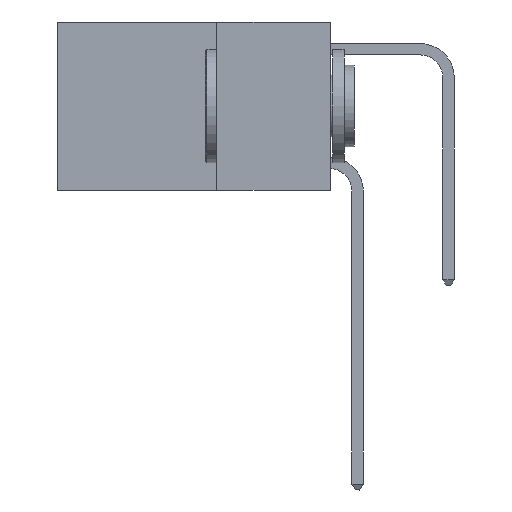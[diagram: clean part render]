
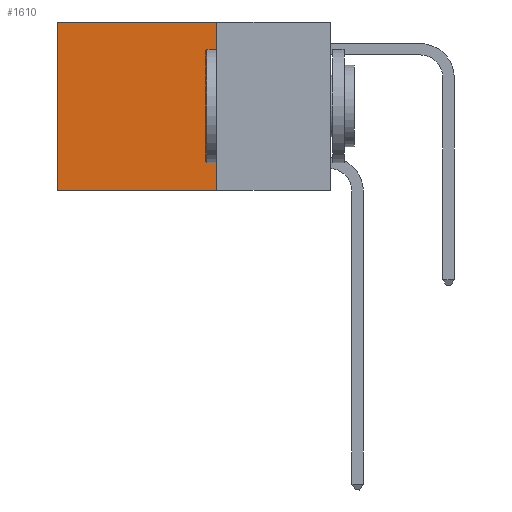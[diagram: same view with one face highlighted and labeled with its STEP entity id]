
A CAD part, left-side view. The second image highlights one B-rep face of the part: STEP entity #1610.
In plain terms, the highlighted planar face has unit normal (-1, 0, 0).
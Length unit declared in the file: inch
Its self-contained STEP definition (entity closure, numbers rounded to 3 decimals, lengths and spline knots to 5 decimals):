
#457 = CARTESIAN_POINT ( 'NONE',  ( 0.2625, 0.25, 0. ) ) ;
#1170 = VECTOR ( 'NONE', #5583, 39.37008 ) ;
#1394 = VERTEX_POINT ( 'NONE', #8471 ) ;
#1610 = ADVANCED_FACE ( 'NONE', ( #7768 ), #3757, .F. ) ;
#2112 = LINE ( 'NONE', #3383, #6817 ) ;
#2234 = VERTEX_POINT ( 'NONE', #4405 ) ;
#2416 = LINE ( 'NONE', #10931, #7415 ) ;
#2614 = CARTESIAN_POINT ( 'NONE',  ( 0.2625, 0.25, -0.37 ) ) ;
#3239 = LINE ( 'NONE', #2614, #11157 ) ;
#3383 = CARTESIAN_POINT ( 'NONE',  ( 0.2625, 0.6, 0. ) ) ;
#3575 = VERTEX_POINT ( 'NONE', #6453 ) ;
#3626 = DIRECTION ( 'NONE',  ( 0., 0., -1. ) ) ;
#3711 = DIRECTION ( 'NONE',  ( 1., 0., 0. ) ) ;
#3733 = CARTESIAN_POINT ( 'NONE',  ( 0.2625, 0.25, 0. ) ) ;
#3740 = CARTESIAN_POINT ( 'NONE',  ( 0.2625, 0.6, 0. ) ) ;
#3757 = PLANE ( 'NONE',  #8220 ) ;
#3978 = EDGE_LOOP ( 'NONE', ( #6916, #9011, #5839, #8820 ) ) ;
#4405 = CARTESIAN_POINT ( 'NONE',  ( 0.2625, 0.25, -0.37 ) ) ;
#4704 = EDGE_CURVE ( 'NONE', #1394, #2234, #11423, .T. ) ;
#4854 = DIRECTION ( 'NONE',  ( 0., 1., 0. ) ) ;
#5583 = DIRECTION ( 'NONE',  ( 0., 0., -1. ) ) ;
#5839 = ORIENTED_EDGE ( 'NONE', *, *, #4704, .F. ) ;
#6453 = CARTESIAN_POINT ( 'NONE',  ( 0.2625, 0.6, -0.37 ) ) ;
#6817 = VECTOR ( 'NONE', #11316, 39.37008 ) ;
#6916 = ORIENTED_EDGE ( 'NONE', *, *, #11519, .T. ) ;
#7415 = VECTOR ( 'NONE', #11876, 39.37008 ) ;
#7768 = FACE_OUTER_BOUND ( 'NONE', #3978, .T. ) ;
#8220 = AXIS2_PLACEMENT_3D ( 'NONE', #3733, #3711, #3626 ) ;
#8471 = CARTESIAN_POINT ( 'NONE',  ( 0.2625, 0.25, 0. ) ) ;
#8820 = ORIENTED_EDGE ( 'NONE', *, *, #11893, .T. ) ;
#9011 = ORIENTED_EDGE ( 'NONE', *, *, #10482, .F. ) ;
#9878 = VERTEX_POINT ( 'NONE', #3740 ) ;
#10482 = EDGE_CURVE ( 'NONE', #2234, #3575, #3239, .T. ) ;
#10931 = CARTESIAN_POINT ( 'NONE',  ( 0.2625, 0.25, 0. ) ) ;
#11157 = VECTOR ( 'NONE', #4854, 39.37008 ) ;
#11316 = DIRECTION ( 'NONE',  ( 0., 0., -1. ) ) ;
#11423 = LINE ( 'NONE', #457, #1170 ) ;
#11519 = EDGE_CURVE ( 'NONE', #9878, #3575, #2112, .T. ) ;
#11876 = DIRECTION ( 'NONE',  ( 0., 1., 0. ) ) ;
#11893 = EDGE_CURVE ( 'NONE', #1394, #9878, #2416, .T. ) ;
